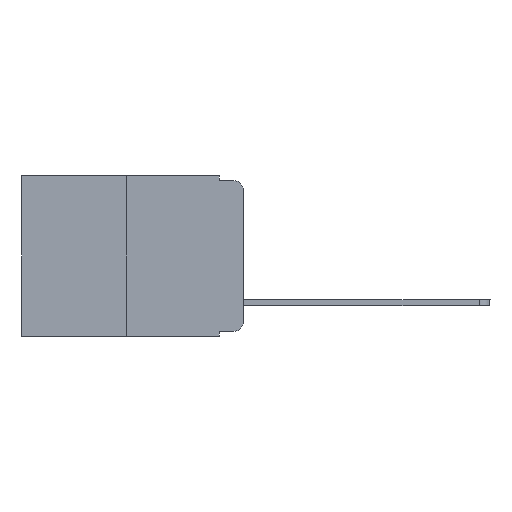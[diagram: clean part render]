
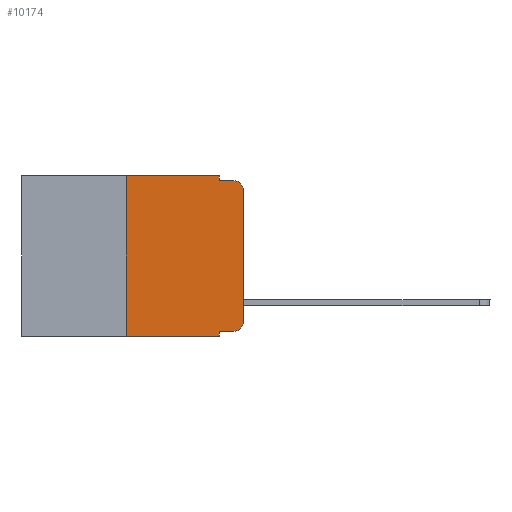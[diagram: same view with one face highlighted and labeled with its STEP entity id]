
A CAD part, left-side view. The second image highlights one B-rep face of the part: STEP entity #10174.
In plain terms, the highlighted planar face has unit normal (-1, 0, 0).
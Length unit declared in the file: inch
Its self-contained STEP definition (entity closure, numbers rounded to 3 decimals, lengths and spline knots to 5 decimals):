
#263 = EDGE_CURVE ( 'NONE', #7784, #9053, #16494, .T. ) ;
#336 = AXIS2_PLACEMENT_3D ( 'NONE', #14360, #7963, #14527 ) ;
#695 = EDGE_LOOP ( 'NONE', ( #2682, #12735, #11022, #15273, #15226, #14318, #11700, #7370, #10288, #12842 ) ) ;
#947 = DIRECTION ( 'NONE',  ( 0., -1., 0. ) ) ;
#1279 = DIRECTION ( 'NONE',  ( 0., 0., 1. ) ) ;
#1362 = LINE ( 'NONE', #1703, #11515 ) ;
#1703 = CARTESIAN_POINT ( 'NONE',  ( 0., 0.473, 0. ) ) ;
#2509 = VERTEX_POINT ( 'NONE', #4070 ) ;
#2682 = ORIENTED_EDGE ( 'NONE', *, *, #6976, .T. ) ;
#2890 = DIRECTION ( 'NONE',  ( 0., -1., 0. ) ) ;
#2993 = VECTOR ( 'NONE', #4422, 39.37008 ) ;
#3289 = EDGE_CURVE ( 'NONE', #15965, #12521, #13889, .T. ) ;
#3694 = DIRECTION ( 'NONE',  ( 0., 0., -1. ) ) ;
#4070 = CARTESIAN_POINT ( 'NONE',  ( 0., 0.25, -0.343 ) ) ;
#4422 = DIRECTION ( 'NONE',  ( 0., 0., 1. ) ) ;
#4472 = VERTEX_POINT ( 'NONE', #16568 ) ;
#4553 = DIRECTION ( 'NONE',  ( 0., 0., -1. ) ) ;
#4745 = EDGE_CURVE ( 'NONE', #15785, #14568, #1362, .T. ) ;
#5129 = EDGE_CURVE ( 'NONE', #12521, #4472, #15613, .T. ) ;
#5404 = CARTESIAN_POINT ( 'NONE',  ( 0., 0.25, 0. ) ) ;
#6173 = EDGE_CURVE ( 'NONE', #14568, #7784, #10154, .T. ) ;
#6260 = VECTOR ( 'NONE', #10258, 39.37008 ) ;
#6805 = CARTESIAN_POINT ( 'NONE',  ( 0., 0.051, -0.01 ) ) ;
#6820 = CARTESIAN_POINT ( 'NONE',  ( 0., 0.051, 0. ) ) ;
#6976 = EDGE_CURVE ( 'NONE', #4472, #12126, #11902, .T. ) ;
#7040 = VECTOR ( 'NONE', #947, 39.37008 ) ;
#7043 = AXIS2_PLACEMENT_3D ( 'NONE', #15535, #7967, #14040 ) ;
#7370 = ORIENTED_EDGE ( 'NONE', *, *, #7744, .F. ) ;
#7744 = EDGE_CURVE ( 'NONE', #15965, #9164, #8463, .T. ) ;
#7784 = VERTEX_POINT ( 'NONE', #9476 ) ;
#7963 = DIRECTION ( 'NONE',  ( 1., 0., 0. ) ) ;
#7967 = DIRECTION ( 'NONE',  ( -1., 0., 0. ) ) ;
#8212 = EDGE_CURVE ( 'NONE', #12126, #9053, #10255, .T. ) ;
#8275 = CARTESIAN_POINT ( 'NONE',  ( 0., 0.051, -0.333 ) ) ;
#8463 = LINE ( 'NONE', #13420, #14278 ) ;
#9053 = VERTEX_POINT ( 'NONE', #9562 ) ;
#9139 = FACE_OUTER_BOUND ( 'NONE', #695, .T. ) ;
#9164 = VERTEX_POINT ( 'NONE', #13682 ) ;
#9476 = CARTESIAN_POINT ( 'NONE',  ( 0., 0.051, -0.01 ) ) ;
#9562 = CARTESIAN_POINT ( 'NONE',  ( 0., 0.02, -0.01 ) ) ;
#9693 = EDGE_CURVE ( 'NONE', #2509, #9164, #10185, .T. ) ;
#9918 = CARTESIAN_POINT ( 'NONE',  ( 0., 0.051, 0. ) ) ;
#10154 = LINE ( 'NONE', #9918, #15315 ) ;
#10174 = ADVANCED_FACE ( 'NONE', ( #9139 ), #13089, .F. ) ;
#10185 = LINE ( 'NONE', #15572, #16214 ) ;
#10255 = CIRCLE ( 'NONE', #15374, 0.02 ) ;
#10258 = DIRECTION ( 'NONE',  ( 0., -1., 0. ) ) ;
#10288 = ORIENTED_EDGE ( 'NONE', *, *, #3289, .T. ) ;
#11022 = ORIENTED_EDGE ( 'NONE', *, *, #263, .F. ) ;
#11459 = VECTOR ( 'NONE', #1279, 39.37008 ) ;
#11515 = VECTOR ( 'NONE', #16059, 39.37008 ) ;
#11700 = ORIENTED_EDGE ( 'NONE', *, *, #9693, .T. ) ;
#11902 = LINE ( 'NONE', #13411, #2993 ) ;
#11994 = DIRECTION ( 'NONE',  ( 0., 0., -1. ) ) ;
#12126 = VERTEX_POINT ( 'NONE', #13685 ) ;
#12214 = CARTESIAN_POINT ( 'NONE',  ( 0., 0.02, -0.03 ) ) ;
#12521 = VERTEX_POINT ( 'NONE', #12558 ) ;
#12558 = CARTESIAN_POINT ( 'NONE',  ( 0., 0.02, -0.333 ) ) ;
#12702 = CARTESIAN_POINT ( 'NONE',  ( 0., 0.051, -0.333 ) ) ;
#12735 = ORIENTED_EDGE ( 'NONE', *, *, #8212, .T. ) ;
#12785 = LINE ( 'NONE', #5404, #11459 ) ;
#12842 = ORIENTED_EDGE ( 'NONE', *, *, #5129, .T. ) ;
#13089 = PLANE ( 'NONE',  #336 ) ;
#13411 = CARTESIAN_POINT ( 'NONE',  ( 0., 0., 0. ) ) ;
#13420 = CARTESIAN_POINT ( 'NONE',  ( 0., 0.051, 0. ) ) ;
#13682 = CARTESIAN_POINT ( 'NONE',  ( 0., 0.051, -0.343 ) ) ;
#13685 = CARTESIAN_POINT ( 'NONE',  ( 0., 0., -0.03 ) ) ;
#13889 = LINE ( 'NONE', #12702, #7040 ) ;
#14040 = DIRECTION ( 'NONE',  ( 0., 0., -1. ) ) ;
#14278 = VECTOR ( 'NONE', #11994, 39.37008 ) ;
#14318 = ORIENTED_EDGE ( 'NONE', *, *, #14415, .F. ) ;
#14348 = CARTESIAN_POINT ( 'NONE',  ( 0., 0.25, 0. ) ) ;
#14360 = CARTESIAN_POINT ( 'NONE',  ( 0., 0.473, 0. ) ) ;
#14415 = EDGE_CURVE ( 'NONE', #2509, #15785, #12785, .T. ) ;
#14527 = DIRECTION ( 'NONE',  ( 0., 0., -1. ) ) ;
#14568 = VERTEX_POINT ( 'NONE', #6820 ) ;
#15226 = ORIENTED_EDGE ( 'NONE', *, *, #4745, .F. ) ;
#15273 = ORIENTED_EDGE ( 'NONE', *, *, #6173, .F. ) ;
#15315 = VECTOR ( 'NONE', #3694, 39.37008 ) ;
#15374 = AXIS2_PLACEMENT_3D ( 'NONE', #12214, #16068, #4553 ) ;
#15535 = CARTESIAN_POINT ( 'NONE',  ( 0., 0.02, -0.313 ) ) ;
#15572 = CARTESIAN_POINT ( 'NONE',  ( 0., 0.473, -0.343 ) ) ;
#15613 = CIRCLE ( 'NONE', #7043, 0.02 ) ;
#15785 = VERTEX_POINT ( 'NONE', #14348 ) ;
#15965 = VERTEX_POINT ( 'NONE', #8275 ) ;
#16059 = DIRECTION ( 'NONE',  ( 0., -1., 0. ) ) ;
#16068 = DIRECTION ( 'NONE',  ( -1., 0., 0. ) ) ;
#16214 = VECTOR ( 'NONE', #2890, 39.37008 ) ;
#16494 = LINE ( 'NONE', #6805, #6260 ) ;
#16568 = CARTESIAN_POINT ( 'NONE',  ( 0., 0., -0.313 ) ) ;
